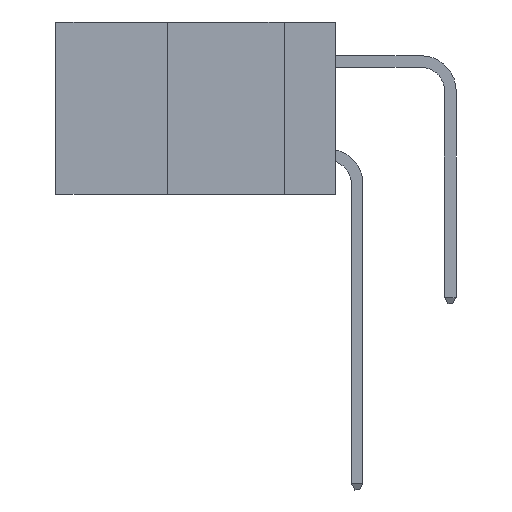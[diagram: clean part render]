
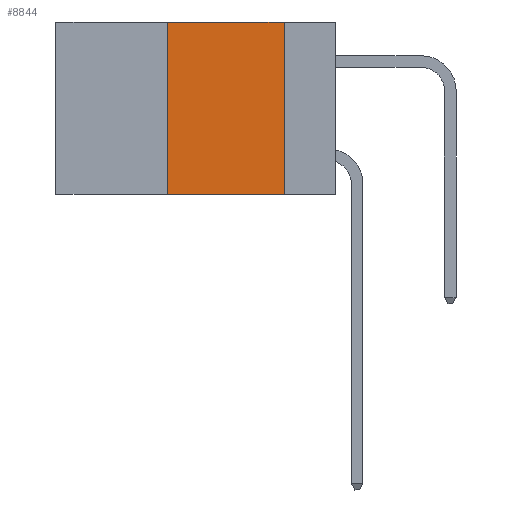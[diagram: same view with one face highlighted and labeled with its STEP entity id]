
A CAD part, left-side view. The second image highlights one B-rep face of the part: STEP entity #8844.
In plain terms, the highlighted planar face has unit normal (-1, 0, 0).
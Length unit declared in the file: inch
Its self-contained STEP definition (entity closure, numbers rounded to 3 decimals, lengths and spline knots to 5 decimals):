
#952 = CARTESIAN_POINT ( 'NONE',  ( 0., 0.36, 0. ) ) ;
#1244 = ORIENTED_EDGE ( 'NONE', *, *, #1806, .T. ) ;
#1806 = EDGE_CURVE ( 'NONE', #15863, #14786, #7616, .T. ) ;
#2152 = CARTESIAN_POINT ( 'NONE',  ( 0., 0.36, -0.37 ) ) ;
#2667 = CARTESIAN_POINT ( 'NONE',  ( 0., 0.6, -0.37 ) ) ;
#2777 = VECTOR ( 'NONE', #13339, 39.37008 ) ;
#3101 = VECTOR ( 'NONE', #24696, 39.37008 ) ;
#5257 = CARTESIAN_POINT ( 'NONE',  ( 0., 0.6, 0. ) ) ;
#5735 = DIRECTION ( 'NONE',  ( 0., 0., -1. ) ) ;
#7379 = CARTESIAN_POINT ( 'NONE',  ( 0., 0.36, 0. ) ) ;
#7616 = LINE ( 'NONE', #2667, #28232 ) ;
#7911 = CARTESIAN_POINT ( 'NONE',  ( 0., 0.6, 0. ) ) ;
#7982 = VERTEX_POINT ( 'NONE', #25454 ) ;
#8844 = ADVANCED_FACE ( 'NONE', ( #12824 ), #27840, .F. ) ;
#11710 = VERTEX_POINT ( 'NONE', #952 ) ;
#12824 = FACE_OUTER_BOUND ( 'NONE', #29999, .T. ) ;
#12913 = EDGE_CURVE ( 'NONE', #7982, #14786, #20739, .T. ) ;
#13339 = DIRECTION ( 'NONE',  ( 0., -1., 0. ) ) ;
#14625 = AXIS2_PLACEMENT_3D ( 'NONE', #5257, #22896, #20411 ) ;
#14786 = VERTEX_POINT ( 'NONE', #30991 ) ;
#15332 = LINE ( 'NONE', #7911, #2777 ) ;
#15863 = VERTEX_POINT ( 'NONE', #2152 ) ;
#17695 = VECTOR ( 'NONE', #5735, 39.37008 ) ;
#17748 = LINE ( 'NONE', #7379, #3101 ) ;
#17855 = ORIENTED_EDGE ( 'NONE', *, *, #31922, .F. ) ;
#18211 = ORIENTED_EDGE ( 'NONE', *, *, #12913, .F. ) ;
#18265 = CARTESIAN_POINT ( 'NONE',  ( 0., 0.11, 0. ) ) ;
#20411 = DIRECTION ( 'NONE',  ( 0., 0., -1. ) ) ;
#20739 = LINE ( 'NONE', #18265, #17695 ) ;
#22896 = DIRECTION ( 'NONE',  ( 1., 0., 0. ) ) ;
#24069 = ORIENTED_EDGE ( 'NONE', *, *, #25865, .F. ) ;
#24696 = DIRECTION ( 'NONE',  ( 0., 0., 1. ) ) ;
#25454 = CARTESIAN_POINT ( 'NONE',  ( 0., 0.11, 0. ) ) ;
#25865 = EDGE_CURVE ( 'NONE', #15863, #11710, #17748, .T. ) ;
#27840 = PLANE ( 'NONE',  #14625 ) ;
#27880 = DIRECTION ( 'NONE',  ( 0., -1., 0. ) ) ;
#28232 = VECTOR ( 'NONE', #27880, 39.37008 ) ;
#29999 = EDGE_LOOP ( 'NONE', ( #18211, #17855, #24069, #1244 ) ) ;
#30991 = CARTESIAN_POINT ( 'NONE',  ( 0., 0.11, -0.37 ) ) ;
#31922 = EDGE_CURVE ( 'NONE', #11710, #7982, #15332, .T. ) ;
